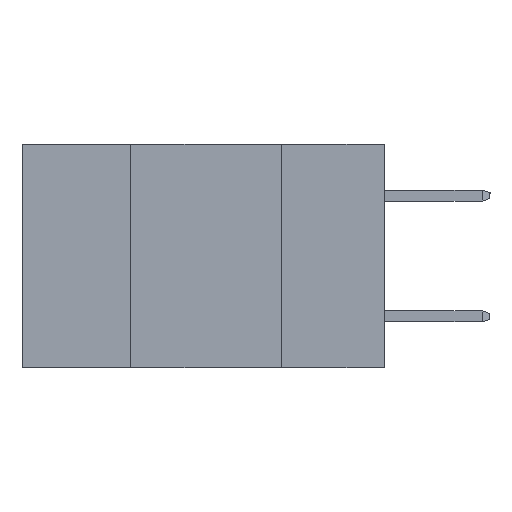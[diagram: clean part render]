
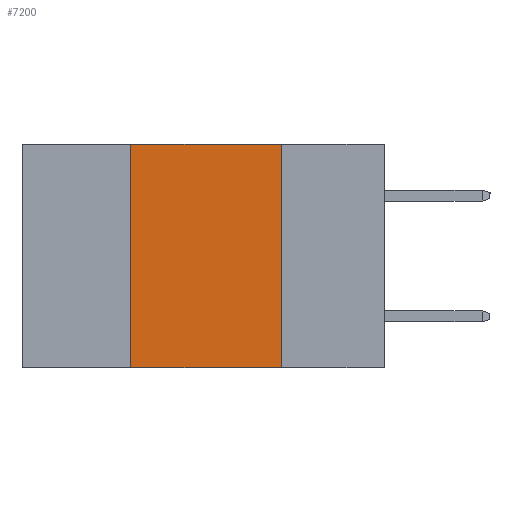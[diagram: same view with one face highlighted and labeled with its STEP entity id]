
A CAD part, left-side view. The second image highlights one B-rep face of the part: STEP entity #7200.
In plain terms, the highlighted planar face has unit normal (-1, 0, 0).
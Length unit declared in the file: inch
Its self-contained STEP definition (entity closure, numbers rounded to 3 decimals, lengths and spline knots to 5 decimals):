
#402 = CARTESIAN_POINT ( 'NONE',  ( 0., 0.17, -0.37 ) ) ;
#423 = PLANE ( 'NONE',  #3500 ) ;
#894 = VECTOR ( 'NONE', #13686, 39.37008 ) ;
#908 = CARTESIAN_POINT ( 'NONE',  ( 0., 0.42, 0. ) ) ;
#1800 = ORIENTED_EDGE ( 'NONE', *, *, #12493, .F. ) ;
#3500 = AXIS2_PLACEMENT_3D ( 'NONE', #7747, #4721, #7959 ) ;
#4555 = DIRECTION ( 'NONE',  ( 0., 0., -1. ) ) ;
#4721 = DIRECTION ( 'NONE',  ( 1., 0., 0. ) ) ;
#5245 = VERTEX_POINT ( 'NONE', #9589 ) ;
#5879 = ORIENTED_EDGE ( 'NONE', *, *, #10783, .F. ) ;
#5883 = EDGE_CURVE ( 'NONE', #5245, #9251, #8991, .T. ) ;
#5925 = DIRECTION ( 'NONE',  ( 0., -1., 0. ) ) ;
#6735 = LINE ( 'NONE', #402, #8985 ) ;
#6773 = ORIENTED_EDGE ( 'NONE', *, *, #6816, .F. ) ;
#6816 = EDGE_CURVE ( 'NONE', #10941, #13265, #8255, .T. ) ;
#6880 = VECTOR ( 'NONE', #5925, 39.37008 ) ;
#7200 = ADVANCED_FACE ( 'NONE', ( #13277 ), #423, .F. ) ;
#7747 = CARTESIAN_POINT ( 'NONE',  ( 0., 0.6, 0. ) ) ;
#7940 = CARTESIAN_POINT ( 'NONE',  ( 0., 0.6, -0.37 ) ) ;
#7959 = DIRECTION ( 'NONE',  ( 0., 0., -1. ) ) ;
#8165 = CARTESIAN_POINT ( 'NONE',  ( 0., 0.42, -0.37 ) ) ;
#8255 = LINE ( 'NONE', #11528, #6880 ) ;
#8985 = VECTOR ( 'NONE', #4555, 39.37008 ) ;
#8991 = LINE ( 'NONE', #7940, #10070 ) ;
#9251 = VERTEX_POINT ( 'NONE', #9837 ) ;
#9589 = CARTESIAN_POINT ( 'NONE',  ( 0., 0.42, -0.37 ) ) ;
#9837 = CARTESIAN_POINT ( 'NONE',  ( 0., 0.17, -0.37 ) ) ;
#10004 = EDGE_LOOP ( 'NONE', ( #1800, #6773, #5879, #10259 ) ) ;
#10070 = VECTOR ( 'NONE', #12691, 39.37008 ) ;
#10259 = ORIENTED_EDGE ( 'NONE', *, *, #5883, .T. ) ;
#10783 = EDGE_CURVE ( 'NONE', #5245, #10941, #11292, .T. ) ;
#10941 = VERTEX_POINT ( 'NONE', #908 ) ;
#11292 = LINE ( 'NONE', #8165, #894 ) ;
#11327 = CARTESIAN_POINT ( 'NONE',  ( 0., 0.17, 0. ) ) ;
#11528 = CARTESIAN_POINT ( 'NONE',  ( 0., 0.6, 0. ) ) ;
#12493 = EDGE_CURVE ( 'NONE', #13265, #9251, #6735, .T. ) ;
#12691 = DIRECTION ( 'NONE',  ( 0., -1., 0. ) ) ;
#13265 = VERTEX_POINT ( 'NONE', #11327 ) ;
#13277 = FACE_OUTER_BOUND ( 'NONE', #10004, .T. ) ;
#13686 = DIRECTION ( 'NONE',  ( 0., 0., 1. ) ) ;
